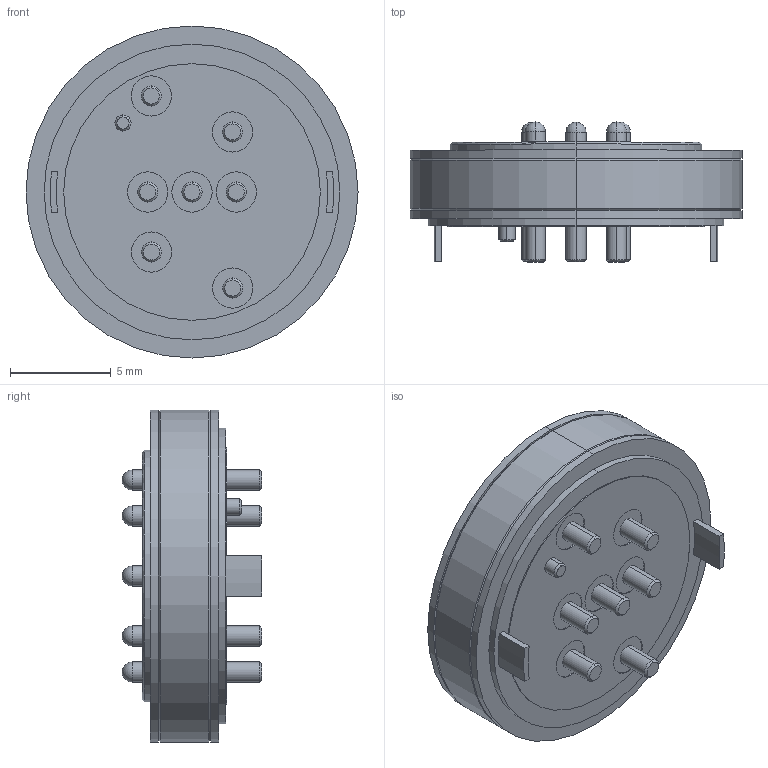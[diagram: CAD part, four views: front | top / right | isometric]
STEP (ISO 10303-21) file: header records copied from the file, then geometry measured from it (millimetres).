
FILE_DESCRIPTION (( 'STEP AP214' ), '1' );
FILE_NAME ('685N05222011G1E.STEP', '2023-05-01T19:12:21', ( '' ), ( '' ), 'SwSTEP 2.0', 'SolidWorks 2020', '' );
FILE_SCHEMA (( 'AUTOMOTIVE_DESIGN' ));
Length unit declared in the file: millimetre
Products named in the file (1): 685N05222011G1E
Bounding box: 16.5 x 6.95 x 16.5 mm (x, y, z)
Volume: 856.1 mm3; surface area: 1563.2 mm2
Topology: 3 solids, 3 shells, 151 faces, 334 edges, 207 vertices
Faces by surface type: cylinder 78, plane 37, cone 22, sphere 14
Entity records: 5723 total; most frequent: DIRECTION 804, CARTESIAN_POINT 651, ORIENTED_EDGE 612, AXIS2_PLACEMENT_3D 346, EDGE_CURVE 306, CIRCLE 194, VERTEX_POINT 193, EDGE_LOOP 183
